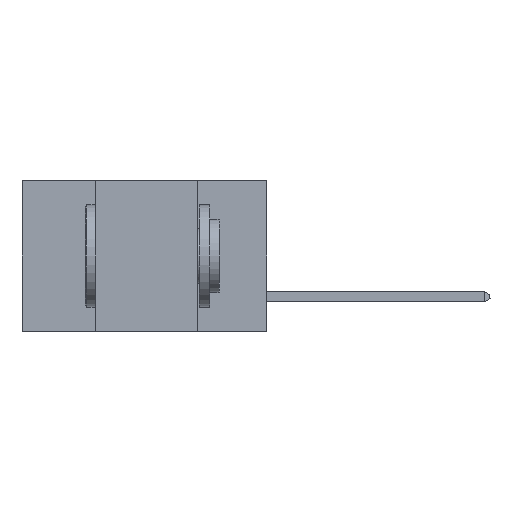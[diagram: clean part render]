
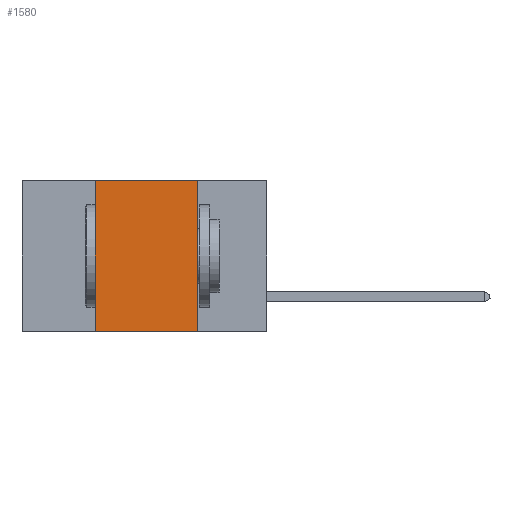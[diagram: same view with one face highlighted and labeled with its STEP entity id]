
A CAD part, left-side view. The second image highlights one B-rep face of the part: STEP entity #1580.
In plain terms, the highlighted planar face has unit normal (-1, 0, 0).
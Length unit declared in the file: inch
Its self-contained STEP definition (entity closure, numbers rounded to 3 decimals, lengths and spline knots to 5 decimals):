
#401 = VECTOR ( 'NONE', #3797, 39.37008 ) ;
#1131 = EDGE_CURVE ( 'NONE', #9912, #16467, #10965, .T. ) ;
#1580 = ADVANCED_FACE ( 'NONE', ( #14466 ), #16923, .F. ) ;
#1675 = ORIENTED_EDGE ( 'NONE', *, *, #11508, .F. ) ;
#1770 = DIRECTION ( 'NONE',  ( 1., 0., 0. ) ) ;
#2276 = CARTESIAN_POINT ( 'NONE',  ( 0., 0.17, 0. ) ) ;
#2926 = DIRECTION ( 'NONE',  ( 0., 0., 1. ) ) ;
#3780 = VERTEX_POINT ( 'NONE', #5470 ) ;
#3797 = DIRECTION ( 'NONE',  ( 0., 0., -1. ) ) ;
#3921 = VECTOR ( 'NONE', #4864, 39.37008 ) ;
#4786 = CARTESIAN_POINT ( 'NONE',  ( 0., 0.17, 0. ) ) ;
#4848 = DIRECTION ( 'NONE',  ( 0., 0., -1. ) ) ;
#4864 = DIRECTION ( 'NONE',  ( 0., -1., 0. ) ) ;
#5236 = LINE ( 'NONE', #17239, #17601 ) ;
#5336 = EDGE_CURVE ( 'NONE', #9663, #3780, #6587, .T. ) ;
#5470 = CARTESIAN_POINT ( 'NONE',  ( 0., 0.42, 0. ) ) ;
#5550 = CARTESIAN_POINT ( 'NONE',  ( 0., 0.17, -0.37 ) ) ;
#6089 = AXIS2_PLACEMENT_3D ( 'NONE', #18394, #1770, #4848 ) ;
#6587 = LINE ( 'NONE', #19396, #17580 ) ;
#6769 = ORIENTED_EDGE ( 'NONE', *, *, #9205, .T. ) ;
#8239 = CARTESIAN_POINT ( 'NONE',  ( 0., 0.42, -0.37 ) ) ;
#8270 = DIRECTION ( 'NONE',  ( 0., -1., 0. ) ) ;
#9205 = EDGE_CURVE ( 'NONE', #9663, #16467, #5236, .T. ) ;
#9663 = VERTEX_POINT ( 'NONE', #8239 ) ;
#9912 = VERTEX_POINT ( 'NONE', #4786 ) ;
#10965 = LINE ( 'NONE', #2276, #401 ) ;
#11508 = EDGE_CURVE ( 'NONE', #3780, #9912, #16623, .T. ) ;
#13948 = EDGE_LOOP ( 'NONE', ( #19362, #1675, #16711, #6769 ) ) ;
#14466 = FACE_OUTER_BOUND ( 'NONE', #13948, .T. ) ;
#16467 = VERTEX_POINT ( 'NONE', #5550 ) ;
#16623 = LINE ( 'NONE', #16813, #3921 ) ;
#16711 = ORIENTED_EDGE ( 'NONE', *, *, #5336, .F. ) ;
#16813 = CARTESIAN_POINT ( 'NONE',  ( 0., 0.6, 0. ) ) ;
#16923 = PLANE ( 'NONE',  #6089 ) ;
#17239 = CARTESIAN_POINT ( 'NONE',  ( 0., 0.6, -0.37 ) ) ;
#17580 = VECTOR ( 'NONE', #2926, 39.37008 ) ;
#17601 = VECTOR ( 'NONE', #8270, 39.37008 ) ;
#18394 = CARTESIAN_POINT ( 'NONE',  ( 0., 0.6, 0. ) ) ;
#19362 = ORIENTED_EDGE ( 'NONE', *, *, #1131, .F. ) ;
#19396 = CARTESIAN_POINT ( 'NONE',  ( 0., 0.42, 0. ) ) ;
